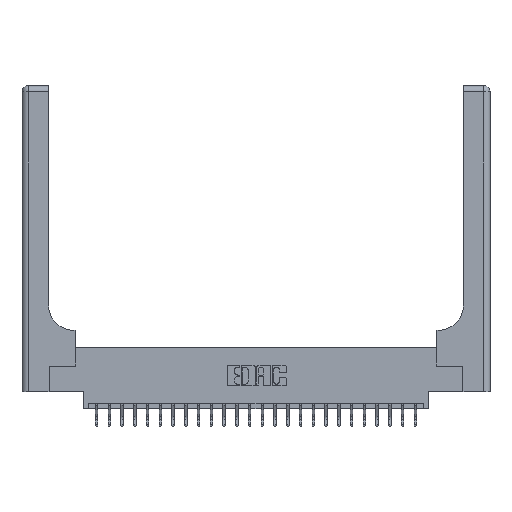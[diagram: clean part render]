
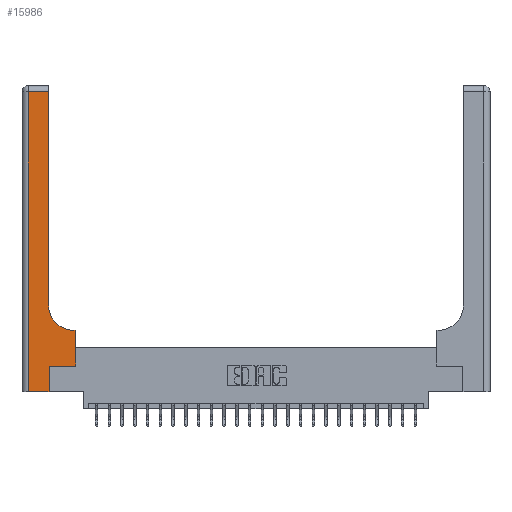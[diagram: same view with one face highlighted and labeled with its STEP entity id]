
A CAD part, top view. The second image highlights one B-rep face of the part: STEP entity #15986.
In plain terms, the highlighted planar face has unit normal (0, 0, 1).
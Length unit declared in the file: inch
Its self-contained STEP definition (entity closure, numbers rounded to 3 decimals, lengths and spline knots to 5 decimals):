
#115 = VERTEX_POINT ( 'NONE', #6221 ) ;
#203 = AXIS2_PLACEMENT_3D ( 'NONE', #14787, #5230, #18590 ) ;
#527 = CARTESIAN_POINT ( 'NONE',  ( 0.26, 0.6, 0.37 ) ) ;
#1294 = VECTOR ( 'NONE', #9852, 39.37008 ) ;
#1427 = DIRECTION ( 'NONE',  ( 0., 1., 0. ) ) ;
#1957 = EDGE_CURVE ( 'NONE', #23636, #9512, #7504, .T. ) ;
#2465 = VERTEX_POINT ( 'NONE', #9803 ) ;
#2494 = DIRECTION ( 'NONE',  ( -1., 0., 0. ) ) ;
#2806 = DIRECTION ( 'NONE',  ( 1., 0., 0. ) ) ;
#3130 = EDGE_LOOP ( 'NONE', ( #9582, #4869, #22602, #3964, #17812, #4269, #22979, #14970, #14951 ) ) ;
#3890 = EDGE_CURVE ( 'NONE', #20810, #5153, #24030, .T. ) ;
#3964 = ORIENTED_EDGE ( 'NONE', *, *, #11430, .T. ) ;
#4269 = ORIENTED_EDGE ( 'NONE', *, *, #23033, .T. ) ;
#4869 = ORIENTED_EDGE ( 'NONE', *, *, #14475, .T. ) ;
#5094 = CARTESIAN_POINT ( 'NONE',  ( 0.26, 0.85, 0.37 ) ) ;
#5101 = DIRECTION ( 'NONE',  ( 0., 0., -1. ) ) ;
#5153 = VERTEX_POINT ( 'NONE', #24158 ) ;
#5230 = DIRECTION ( 'NONE',  ( 0., 0., -1. ) ) ;
#5540 = VECTOR ( 'NONE', #15045, 39.37008 ) ;
#5823 = CIRCLE ( 'NONE', #24258, 0.25 ) ;
#6221 = CARTESIAN_POINT ( 'NONE',  ( 0.265, 0., 0.37 ) ) ;
#6258 = CARTESIAN_POINT ( 'NONE',  ( 0.528, 0.6, 0.37 ) ) ;
#6384 = CARTESIAN_POINT ( 'NONE',  ( 0., 2.94, 0.37 ) ) ;
#7504 = LINE ( 'NONE', #527, #22042 ) ;
#7832 = VERTEX_POINT ( 'NONE', #24086 ) ;
#8233 = DIRECTION ( 'NONE',  ( -1., 0., 0. ) ) ;
#8240 = CARTESIAN_POINT ( 'NONE',  ( 0.51, 0.6, 0.37 ) ) ;
#8981 = VECTOR ( 'NONE', #18143, 39.37008 ) ;
#8988 = VERTEX_POINT ( 'NONE', #19868 ) ;
#9290 = VERTEX_POINT ( 'NONE', #24355 ) ;
#9512 = VERTEX_POINT ( 'NONE', #8240 ) ;
#9582 = ORIENTED_EDGE ( 'NONE', *, *, #3890, .T. ) ;
#9803 = CARTESIAN_POINT ( 'NONE',  ( 0.06, 2.94, 0.37 ) ) ;
#9852 = DIRECTION ( 'NONE',  ( 0., -1., 0. ) ) ;
#11256 = LINE ( 'NONE', #16957, #5540 ) ;
#11379 = EDGE_CURVE ( 'NONE', #115, #7832, #21295, .T. ) ;
#11430 = EDGE_CURVE ( 'NONE', #8988, #115, #11256, .T. ) ;
#11543 = LINE ( 'NONE', #19225, #1294 ) ;
#11619 = EDGE_CURVE ( 'NONE', #2465, #8988, #11543, .T. ) ;
#11761 = VECTOR ( 'NONE', #2494, 39.37008 ) ;
#11960 = LINE ( 'NONE', #15623, #20211 ) ;
#13354 = VECTOR ( 'NONE', #2806, 39.37008 ) ;
#13730 = DIRECTION ( 'NONE',  ( 0., 1., 0. ) ) ;
#14475 = EDGE_CURVE ( 'NONE', #5153, #2465, #16830, .T. ) ;
#14718 = FACE_OUTER_BOUND ( 'NONE', #3130, .T. ) ;
#14787 = CARTESIAN_POINT ( 'NONE',  ( 0., 3., 0.37 ) ) ;
#14881 = CARTESIAN_POINT ( 'NONE',  ( 0.265, 0., 0.37 ) ) ;
#14951 = ORIENTED_EDGE ( 'NONE', *, *, #23160, .T. ) ;
#14970 = ORIENTED_EDGE ( 'NONE', *, *, #1957, .T. ) ;
#15045 = DIRECTION ( 'NONE',  ( 1., 0., 0. ) ) ;
#15623 = CARTESIAN_POINT ( 'NONE',  ( 0.528, 0.25, 0.37 ) ) ;
#15986 = ADVANCED_FACE ( 'NONE', ( #14718 ), #22242, .F. ) ;
#16339 = VECTOR ( 'NONE', #1427, 39.37008 ) ;
#16578 = CARTESIAN_POINT ( 'NONE',  ( 0.51, 0.85, 0.37 ) ) ;
#16830 = LINE ( 'NONE', #6384, #11761 ) ;
#16957 = CARTESIAN_POINT ( 'NONE',  ( 0., 0., 0.37 ) ) ;
#17812 = ORIENTED_EDGE ( 'NONE', *, *, #11379, .T. ) ;
#18143 = DIRECTION ( 'NONE',  ( 0., 1., 0. ) ) ;
#18386 = LINE ( 'NONE', #21802, #13354 ) ;
#18467 = DIRECTION ( 'NONE',  ( 1., 0., 0. ) ) ;
#18590 = DIRECTION ( 'NONE',  ( -1., 0., 0. ) ) ;
#19225 = CARTESIAN_POINT ( 'NONE',  ( 0.06, 3., 0.37 ) ) ;
#19868 = CARTESIAN_POINT ( 'NONE',  ( 0.06, 0., 0.37 ) ) ;
#19995 = CARTESIAN_POINT ( 'NONE',  ( 0.26, 3., 0.37 ) ) ;
#20211 = VECTOR ( 'NONE', #13730, 39.37008 ) ;
#20810 = VERTEX_POINT ( 'NONE', #5094 ) ;
#21085 = EDGE_CURVE ( 'NONE', #9290, #23636, #11960, .T. ) ;
#21295 = LINE ( 'NONE', #14881, #16339 ) ;
#21802 = CARTESIAN_POINT ( 'NONE',  ( 0.265, 0.25, 0.37 ) ) ;
#22042 = VECTOR ( 'NONE', #8233, 39.37008 ) ;
#22242 = PLANE ( 'NONE',  #203 ) ;
#22602 = ORIENTED_EDGE ( 'NONE', *, *, #11619, .T. ) ;
#22979 = ORIENTED_EDGE ( 'NONE', *, *, #21085, .T. ) ;
#23033 = EDGE_CURVE ( 'NONE', #7832, #9290, #18386, .T. ) ;
#23160 = EDGE_CURVE ( 'NONE', #9512, #20810, #5823, .T. ) ;
#23636 = VERTEX_POINT ( 'NONE', #6258 ) ;
#24030 = LINE ( 'NONE', #19995, #8981 ) ;
#24086 = CARTESIAN_POINT ( 'NONE',  ( 0.265, 0.25, 0.37 ) ) ;
#24158 = CARTESIAN_POINT ( 'NONE',  ( 0.26, 2.94, 0.37 ) ) ;
#24258 = AXIS2_PLACEMENT_3D ( 'NONE', #16578, #5101, #18467 ) ;
#24355 = CARTESIAN_POINT ( 'NONE',  ( 0.528, 0.25, 0.37 ) ) ;
